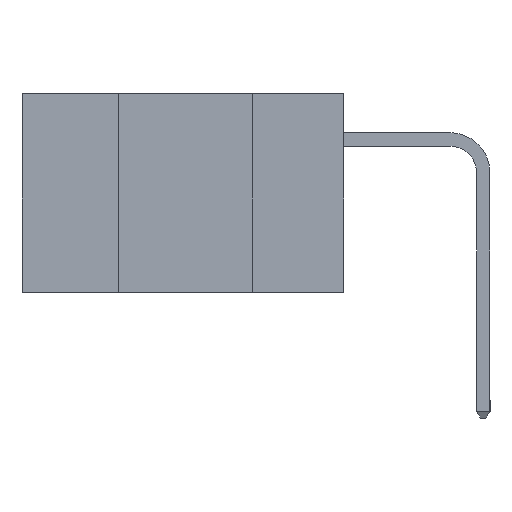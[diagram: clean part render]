
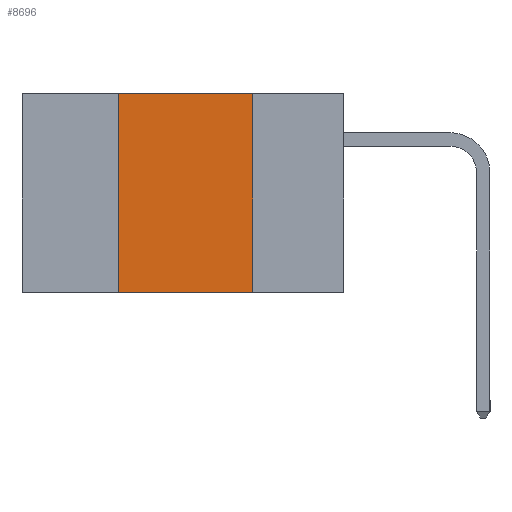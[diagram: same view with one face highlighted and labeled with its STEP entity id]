
A CAD part, left-side view. The second image highlights one B-rep face of the part: STEP entity #8696.
In plain terms, the highlighted planar face has unit normal (-1, 0, 0).
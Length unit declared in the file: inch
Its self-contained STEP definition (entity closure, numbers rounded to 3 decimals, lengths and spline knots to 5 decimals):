
#261 = FACE_OUTER_BOUND ( 'NONE', #11355, .T. ) ;
#495 = CARTESIAN_POINT ( 'NONE',  ( 0., 0.17, -0.37 ) ) ;
#2613 = CARTESIAN_POINT ( 'NONE',  ( 0., 0.17, 0. ) ) ;
#2953 = LINE ( 'NONE', #4871, #21971 ) ;
#3207 = CARTESIAN_POINT ( 'NONE',  ( 0., 0.17, -0.37 ) ) ;
#3526 = VERTEX_POINT ( 'NONE', #20734 ) ;
#4312 = LINE ( 'NONE', #19710, #13591 ) ;
#4433 = DIRECTION ( 'NONE',  ( 0., -1., 0. ) ) ;
#4493 = LINE ( 'NONE', #3207, #16073 ) ;
#4871 = CARTESIAN_POINT ( 'NONE',  ( 0., 0.6, 0. ) ) ;
#4873 = ORIENTED_EDGE ( 'NONE', *, *, #6992, .T. ) ;
#5747 = VECTOR ( 'NONE', #10055, 39.37008 ) ;
#6992 = EDGE_CURVE ( 'NONE', #3526, #16323, #4312, .T. ) ;
#7021 = DIRECTION ( 'NONE',  ( 0., 0., -1. ) ) ;
#7445 = ORIENTED_EDGE ( 'NONE', *, *, #9605, .F. ) ;
#8696 = ADVANCED_FACE ( 'NONE', ( #261 ), #15022, .F. ) ;
#9253 = ORIENTED_EDGE ( 'NONE', *, *, #17772, .F. ) ;
#9605 = EDGE_CURVE ( 'NONE', #20724, #10683, #2953, .T. ) ;
#10055 = DIRECTION ( 'NONE',  ( 0., 0., 1. ) ) ;
#10683 = VERTEX_POINT ( 'NONE', #2613 ) ;
#11355 = EDGE_LOOP ( 'NONE', ( #12077, #7445, #9253, #4873 ) ) ;
#12077 = ORIENTED_EDGE ( 'NONE', *, *, #18682, .F. ) ;
#13591 = VECTOR ( 'NONE', #15178, 39.37008 ) ;
#14969 = DIRECTION ( 'NONE',  ( 0., 0., -1. ) ) ;
#14973 = DIRECTION ( 'NONE',  ( 1., 0., 0. ) ) ;
#15022 = PLANE ( 'NONE',  #20227 ) ;
#15178 = DIRECTION ( 'NONE',  ( 0., -1., 0. ) ) ;
#15182 = CARTESIAN_POINT ( 'NONE',  ( 0., 0.6, 0. ) ) ;
#15555 = LINE ( 'NONE', #19186, #5747 ) ;
#16073 = VECTOR ( 'NONE', #7021, 39.37008 ) ;
#16323 = VERTEX_POINT ( 'NONE', #495 ) ;
#17772 = EDGE_CURVE ( 'NONE', #3526, #20724, #15555, .T. ) ;
#18682 = EDGE_CURVE ( 'NONE', #10683, #16323, #4493, .T. ) ;
#19186 = CARTESIAN_POINT ( 'NONE',  ( 0., 0.42, -0.37 ) ) ;
#19450 = CARTESIAN_POINT ( 'NONE',  ( 0., 0.42, 0. ) ) ;
#19710 = CARTESIAN_POINT ( 'NONE',  ( 0., 0.6, -0.37 ) ) ;
#20227 = AXIS2_PLACEMENT_3D ( 'NONE', #15182, #14973, #14969 ) ;
#20724 = VERTEX_POINT ( 'NONE', #19450 ) ;
#20734 = CARTESIAN_POINT ( 'NONE',  ( 0., 0.42, -0.37 ) ) ;
#21971 = VECTOR ( 'NONE', #4433, 39.37008 ) ;
